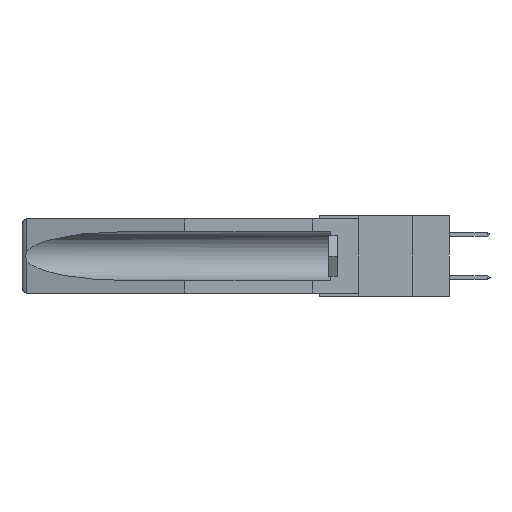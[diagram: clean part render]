
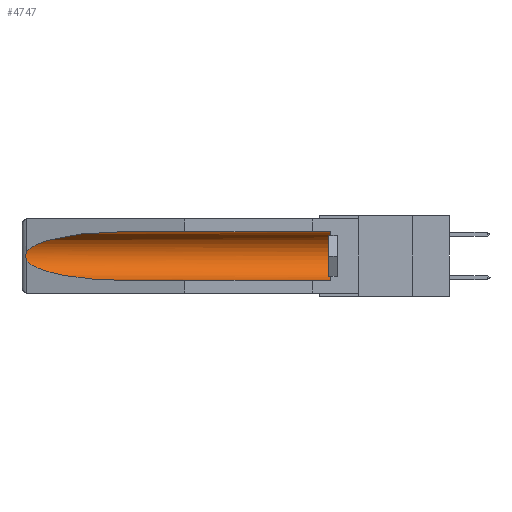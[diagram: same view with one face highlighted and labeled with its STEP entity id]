
A CAD part, left-side view. The second image highlights one B-rep face of the part: STEP entity #4747.
In plain terms, the highlighted cylindrical face has radius 2.857 mm (diameter 5.715 mm), a partial arc.
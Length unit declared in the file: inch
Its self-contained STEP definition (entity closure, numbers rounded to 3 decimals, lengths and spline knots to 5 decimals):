
#105 = ORIENTED_EDGE ( 'NONE', *, *, #3798, .T. ) ;
#841 = VERTEX_POINT ( 'NONE', #8930 ) ;
#1642 = CARTESIAN_POINT ( 'NONE',  ( 0.21114, 1.30732, -0.284 ) ) ;
#1742 = LINE ( 'NONE', #14494, #13031 ) ;
#1761 = VERTEX_POINT ( 'NONE', #14717 ) ;
#1782 = CARTESIAN_POINT ( 'NONE',  ( 0.155, 1.07973, -0.284 ) ) ;
#1868 = VERTEX_POINT ( 'NONE', #1782 ) ;
#3028 = AXIS2_PLACEMENT_3D ( 'NONE', #7701, #5231, #7640 ) ;
#3286 = VERTEX_POINT ( 'NONE', #6060 ) ;
#3335 = CARTESIAN_POINT ( 'NONE',  ( 0.155, 0.126, -0.1715 ) ) ;
#3486 = ORIENTED_EDGE ( 'NONE', *, *, #15223, .F. ) ;
#3542 = VERTEX_POINT ( 'NONE', #10873 ) ;
#3569 = CARTESIAN_POINT ( 'NONE',  ( 0.21114, 1.30732, -0.059 ) ) ;
#3798 = EDGE_CURVE ( 'NONE', #3286, #1868, #13923, .T. ) ;
#3952 = ORIENTED_EDGE ( 'NONE', *, *, #10995, .T. ) ;
#4528 = EDGE_CURVE ( 'NONE', #841, #3542, #13508, .T. ) ;
#4747 = ADVANCED_FACE ( 'NONE', ( #15662 ), #7520, .F. ) ;
#5197 = CARTESIAN_POINT ( 'NONE',  ( 0.25451, 1.48313, -0.24835 ) ) ;
#5231 = DIRECTION ( 'NONE',  ( 0., 1., 0. ) ) ;
#6060 = CARTESIAN_POINT ( 'NONE',  ( 0.26537, 1.52718, -0.19328 ) ) ;
#6535 = ORIENTED_EDGE ( 'NONE', *, *, #4528, .T. ) ;
#6598 = CARTESIAN_POINT ( 'NONE',  ( 0.2675, 1.53308, -0.17534 ) ) ;
#6876 = DIRECTION ( 'NONE',  ( 0., 0., 1. ) ) ;
#7022 =( BOUNDED_CURVE ( )  B_SPLINE_CURVE ( 3, ( #8385, #3569, #7451, #11146 ),
 .UNSPECIFIED., .F., .F. ) 
 B_SPLINE_CURVE_WITH_KNOTS ( ( 4, 4 ),
 ( 4.71239, 6.08839 ),
 .UNSPECIFIED. ) 
 CURVE ( )  GEOMETRIC_REPRESENTATION_ITEM ( )  RATIONAL_B_SPLINE_CURVE ( ( 1., 0.848, 0.848, 1. ) ) 
 REPRESENTATION_ITEM ( '' )  );
#7451 = CARTESIAN_POINT ( 'NONE',  ( 0.25451, 1.48313, -0.09465 ) ) ;
#7512 = CARTESIAN_POINT ( 'NONE',  ( 0.26597, 1.52961, -0.15275 ) ) ;
#7520 = CYLINDRICAL_SURFACE ( 'NONE', #3028, 0.1125 ) ;
#7535 = VECTOR ( 'NONE', #13981, 39.37008 ) ;
#7565 = CARTESIAN_POINT ( 'NONE',  ( 0.26654, 1.53092, -0.15636 ) ) ;
#7618 = CARTESIAN_POINT ( 'NONE',  ( 0.26537, 1.52718, -0.19328 ) ) ;
#7640 = DIRECTION ( 'NONE',  ( 0., 0., 1. ) ) ;
#7701 = CARTESIAN_POINT ( 'NONE',  ( 0.155, -0.30754, -0.1715 ) ) ;
#7722 = CARTESIAN_POINT ( 'NONE',  ( 0.26537, 1.52718, -0.19328 ) ) ;
#8195 = DIRECTION ( 'NONE',  ( 0., -1., 0. ) ) ;
#8385 = CARTESIAN_POINT ( 'NONE',  ( 0.155, 1.07973, -0.059 ) ) ;
#8440 = B_SPLINE_CURVE_WITH_KNOTS ( 'NONE', 3,
 ( #14974, #7512, #7565, #10037, #14742, #6598, #10295, #13738, #13945, #7618 ),
 .UNSPECIFIED., .F., .F.,
 ( 4, 2, 2, 2, 4 ),
 ( 0., 0.00029, 0.00058, 0.00087, 0.00117 ),
 .UNSPECIFIED. ) ;
#8711 = ORIENTED_EDGE ( 'NONE', *, *, #8944, .T. ) ;
#8930 = CARTESIAN_POINT ( 'NONE',  ( 0.155, 0.126, -0.059 ) ) ;
#8944 = EDGE_CURVE ( 'NONE', #1761, #841, #9128, .T. ) ;
#9128 = CIRCLE ( 'NONE', #9579, 0.1125 ) ;
#9579 = AXIS2_PLACEMENT_3D ( 'NONE', #3335, #8195, #6876 ) ;
#10037 = CARTESIAN_POINT ( 'NONE',  ( 0.2673, 1.5327, -0.16383 ) ) ;
#10295 = CARTESIAN_POINT ( 'NONE',  ( 0.2673, 1.53269, -0.17917 ) ) ;
#10594 = DIRECTION ( 'NONE',  ( 0., 1., 0. ) ) ;
#10873 = CARTESIAN_POINT ( 'NONE',  ( 0.155, 1.07973, -0.059 ) ) ;
#10995 = EDGE_CURVE ( 'NONE', #3542, #11118, #7022, .T. ) ;
#11118 = VERTEX_POINT ( 'NONE', #13983 ) ;
#11146 = CARTESIAN_POINT ( 'NONE',  ( 0.26537, 1.52718, -0.14972 ) ) ;
#13018 = EDGE_LOOP ( 'NONE', ( #3952, #14542, #105, #3486, #8711, #6535 ) ) ;
#13031 = VECTOR ( 'NONE', #10594, 39.37008 ) ;
#13474 = EDGE_CURVE ( 'NONE', #11118, #3286, #8440, .T. ) ;
#13508 = LINE ( 'NONE', #15228, #7535 ) ;
#13738 = CARTESIAN_POINT ( 'NONE',  ( 0.26655, 1.53094, -0.18657 ) ) ;
#13923 =( BOUNDED_CURVE ( )  B_SPLINE_CURVE ( 3, ( #7722, #5197, #1642, #15180 ),
 .UNSPECIFIED., .F., .F. ) 
 B_SPLINE_CURVE_WITH_KNOTS ( ( 4, 4 ),
 ( 0.1948, 1.5708 ),
 .UNSPECIFIED. ) 
 CURVE ( )  GEOMETRIC_REPRESENTATION_ITEM ( )  RATIONAL_B_SPLINE_CURVE ( ( 1., 0.848, 0.848, 1. ) ) 
 REPRESENTATION_ITEM ( '' )  );
#13945 = CARTESIAN_POINT ( 'NONE',  ( 0.26597, 1.5296, -0.19026 ) ) ;
#13981 = DIRECTION ( 'NONE',  ( 0., 1., 0. ) ) ;
#13983 = CARTESIAN_POINT ( 'NONE',  ( 0.26537, 1.52718, -0.14972 ) ) ;
#14494 = CARTESIAN_POINT ( 'NONE',  ( 0.155, -0.30754, -0.284 ) ) ;
#14542 = ORIENTED_EDGE ( 'NONE', *, *, #13474, .T. ) ;
#14717 = CARTESIAN_POINT ( 'NONE',  ( 0.155, 0.126, -0.284 ) ) ;
#14742 = CARTESIAN_POINT ( 'NONE',  ( 0.2675, 1.53308, -0.16763 ) ) ;
#14974 = CARTESIAN_POINT ( 'NONE',  ( 0.26537, 1.52718, -0.14972 ) ) ;
#15180 = CARTESIAN_POINT ( 'NONE',  ( 0.155, 1.07973, -0.284 ) ) ;
#15223 = EDGE_CURVE ( 'NONE', #1761, #1868, #1742, .T. ) ;
#15228 = CARTESIAN_POINT ( 'NONE',  ( 0.155, -0.30754, -0.059 ) ) ;
#15662 = FACE_OUTER_BOUND ( 'NONE', #13018, .T. ) ;
